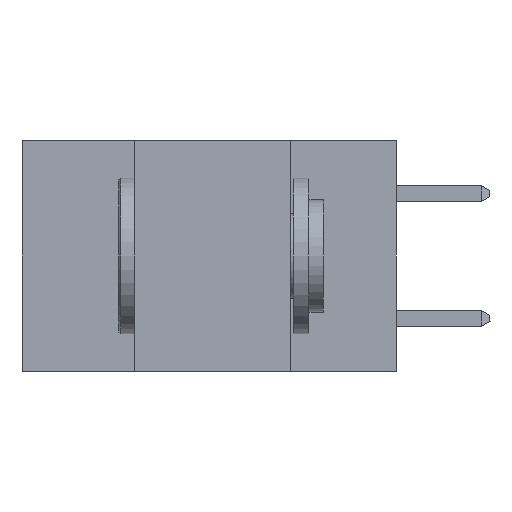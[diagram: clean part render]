
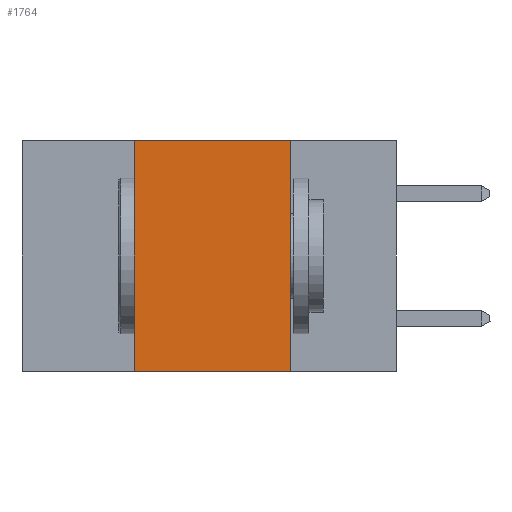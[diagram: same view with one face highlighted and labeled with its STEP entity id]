
A CAD part, left-side view. The second image highlights one B-rep face of the part: STEP entity #1764.
In plain terms, the highlighted planar face has unit normal (-1, 0, 0).
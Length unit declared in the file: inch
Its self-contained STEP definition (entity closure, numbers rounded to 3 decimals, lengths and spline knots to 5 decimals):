
#104 = ORIENTED_EDGE ( 'NONE', *, *, #2415, .F. ) ;
#178 = PLANE ( 'NONE',  #4238 ) ;
#348 = CARTESIAN_POINT ( 'NONE',  ( 0., 0.17, 0. ) ) ;
#1335 = LINE ( 'NONE', #348, #10043 ) ;
#1496 = VERTEX_POINT ( 'NONE', #8496 ) ;
#1764 = ADVANCED_FACE ( 'NONE', ( #4225 ), #178, .F. ) ;
#1908 = DIRECTION ( 'NONE',  ( 0., 0., 1. ) ) ;
#2022 = VECTOR ( 'NONE', #4557, 39.37008 ) ;
#2155 = LINE ( 'NONE', #9371, #11241 ) ;
#2415 = EDGE_CURVE ( 'NONE', #9202, #5105, #4618, .T. ) ;
#3731 = CARTESIAN_POINT ( 'NONE',  ( 0., 0.42, 0. ) ) ;
#4183 = VECTOR ( 'NONE', #1908, 39.37008 ) ;
#4225 = FACE_OUTER_BOUND ( 'NONE', #6931, .T. ) ;
#4238 = AXIS2_PLACEMENT_3D ( 'NONE', #5292, #9200, #9951 ) ;
#4557 = DIRECTION ( 'NONE',  ( 0., -1., 0. ) ) ;
#4618 = LINE ( 'NONE', #9108, #2022 ) ;
#5074 = ORIENTED_EDGE ( 'NONE', *, *, #9145, .F. ) ;
#5105 = VERTEX_POINT ( 'NONE', #8995 ) ;
#5292 = CARTESIAN_POINT ( 'NONE',  ( 0., 0.6, 0. ) ) ;
#5825 = VERTEX_POINT ( 'NONE', #6531 ) ;
#6438 = DIRECTION ( 'NONE',  ( 0., 0., -1. ) ) ;
#6531 = CARTESIAN_POINT ( 'NONE',  ( 0., 0.42, -0.37 ) ) ;
#6931 = EDGE_LOOP ( 'NONE', ( #9574, #104, #5074, #10846 ) ) ;
#7740 = EDGE_CURVE ( 'NONE', #5105, #1496, #1335, .T. ) ;
#8446 = DIRECTION ( 'NONE',  ( 0., -1., 0. ) ) ;
#8496 = CARTESIAN_POINT ( 'NONE',  ( 0., 0.17, -0.37 ) ) ;
#8846 = EDGE_CURVE ( 'NONE', #5825, #1496, #2155, .T. ) ;
#8995 = CARTESIAN_POINT ( 'NONE',  ( 0., 0.17, 0. ) ) ;
#9108 = CARTESIAN_POINT ( 'NONE',  ( 0., 0.6, 0. ) ) ;
#9145 = EDGE_CURVE ( 'NONE', #5825, #9202, #11230, .T. ) ;
#9200 = DIRECTION ( 'NONE',  ( 1., 0., 0. ) ) ;
#9202 = VERTEX_POINT ( 'NONE', #3731 ) ;
#9371 = CARTESIAN_POINT ( 'NONE',  ( 0., 0.6, -0.37 ) ) ;
#9574 = ORIENTED_EDGE ( 'NONE', *, *, #7740, .F. ) ;
#9951 = DIRECTION ( 'NONE',  ( 0., 0., -1. ) ) ;
#10043 = VECTOR ( 'NONE', #6438, 39.37008 ) ;
#10846 = ORIENTED_EDGE ( 'NONE', *, *, #8846, .T. ) ;
#11230 = LINE ( 'NONE', #11346, #4183 ) ;
#11241 = VECTOR ( 'NONE', #8446, 39.37008 ) ;
#11346 = CARTESIAN_POINT ( 'NONE',  ( 0., 0.42, 0. ) ) ;
